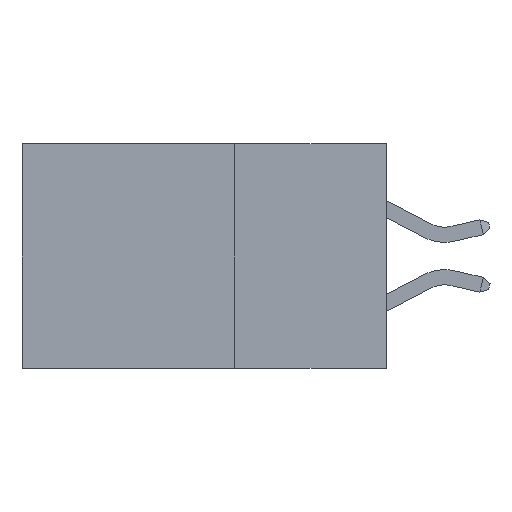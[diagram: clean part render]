
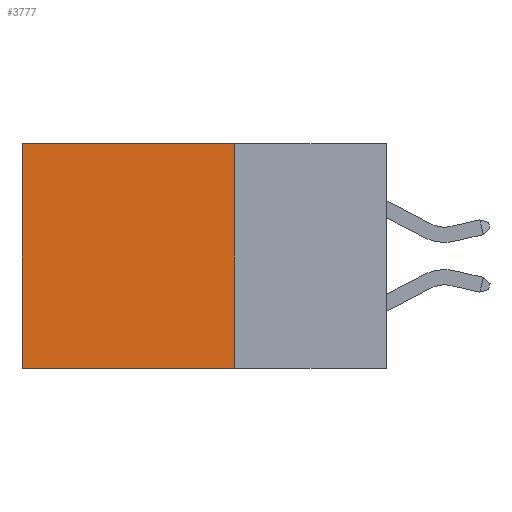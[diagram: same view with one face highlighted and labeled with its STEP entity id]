
A CAD part, left-side view. The second image highlights one B-rep face of the part: STEP entity #3777.
In plain terms, the highlighted planar face has unit normal (-1, 0, 0).
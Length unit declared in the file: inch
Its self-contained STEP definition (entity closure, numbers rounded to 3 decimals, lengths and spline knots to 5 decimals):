
#947 = ORIENTED_EDGE ( 'NONE', *, *, #3785, .T. ) ;
#2215 = VERTEX_POINT ( 'NONE', #11274 ) ;
#2335 = VECTOR ( 'NONE', #4762, 39.37008 ) ;
#2712 = VECTOR ( 'NONE', #16402, 39.37008 ) ;
#2849 = CARTESIAN_POINT ( 'NONE',  ( 0.2615, 0.25, -0.37 ) ) ;
#2950 = CARTESIAN_POINT ( 'NONE',  ( 0.2615, 0.25, 0. ) ) ;
#3107 = LINE ( 'NONE', #20699, #12787 ) ;
#3777 = ADVANCED_FACE ( 'NONE', ( #7632 ), #20957, .F. ) ;
#3785 = EDGE_CURVE ( 'NONE', #2215, #20115, #3107, .T. ) ;
#4239 = ORIENTED_EDGE ( 'NONE', *, *, #15426, .F. ) ;
#4762 = DIRECTION ( 'NONE',  ( 0., 1., 0. ) ) ;
#5594 = ORIENTED_EDGE ( 'NONE', *, *, #9920, .T. ) ;
#7224 = EDGE_LOOP ( 'NONE', ( #947, #19098, #4239, #5594 ) ) ;
#7632 = FACE_OUTER_BOUND ( 'NONE', #7224, .T. ) ;
#9920 = EDGE_CURVE ( 'NONE', #23022, #2215, #13567, .T. ) ;
#11274 = CARTESIAN_POINT ( 'NONE',  ( 0.2615, 0.6, 0. ) ) ;
#12787 = VECTOR ( 'NONE', #21012, 39.37008 ) ;
#13335 = LINE ( 'NONE', #22018, #22784 ) ;
#13567 = LINE ( 'NONE', #2950, #2712 ) ;
#13905 = VERTEX_POINT ( 'NONE', #23553 ) ;
#15204 = CARTESIAN_POINT ( 'NONE',  ( 0.2615, 0.6, -0.37 ) ) ;
#15426 = EDGE_CURVE ( 'NONE', #23022, #13905, #13335, .T. ) ;
#16402 = DIRECTION ( 'NONE',  ( 0., 1., 0. ) ) ;
#17651 = LINE ( 'NONE', #2849, #2335 ) ;
#18106 = EDGE_CURVE ( 'NONE', #13905, #20115, #17651, .T. ) ;
#19098 = ORIENTED_EDGE ( 'NONE', *, *, #18106, .F. ) ;
#19272 = AXIS2_PLACEMENT_3D ( 'NONE', #20800, #20747, #20724 ) ;
#20115 = VERTEX_POINT ( 'NONE', #15204 ) ;
#20699 = CARTESIAN_POINT ( 'NONE',  ( 0.2615, 0.6, -0.37 ) ) ;
#20724 = DIRECTION ( 'NONE',  ( 0., 0., -1. ) ) ;
#20747 = DIRECTION ( 'NONE',  ( 1., 0., 0. ) ) ;
#20800 = CARTESIAN_POINT ( 'NONE',  ( 0.2615, 0.25, -0.37 ) ) ;
#20957 = PLANE ( 'NONE',  #19272 ) ;
#21012 = DIRECTION ( 'NONE',  ( 0., 0., -1. ) ) ;
#22018 = CARTESIAN_POINT ( 'NONE',  ( 0.2615, 0.25, -0.37 ) ) ;
#22784 = VECTOR ( 'NONE', #23875, 39.37008 ) ;
#23022 = VERTEX_POINT ( 'NONE', #23737 ) ;
#23553 = CARTESIAN_POINT ( 'NONE',  ( 0.2615, 0.25, -0.37 ) ) ;
#23737 = CARTESIAN_POINT ( 'NONE',  ( 0.2615, 0.25, 0. ) ) ;
#23875 = DIRECTION ( 'NONE',  ( 0., 0., -1. ) ) ;
